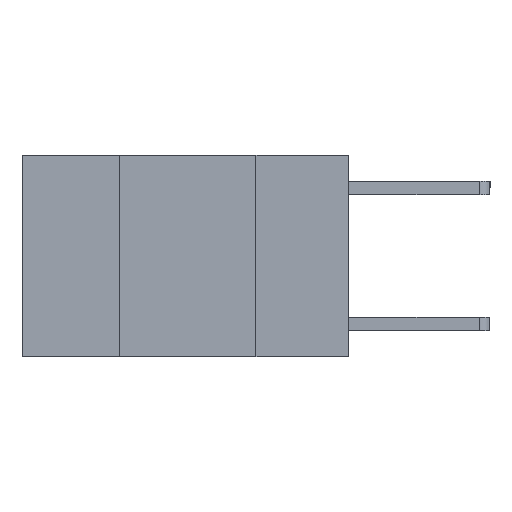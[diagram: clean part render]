
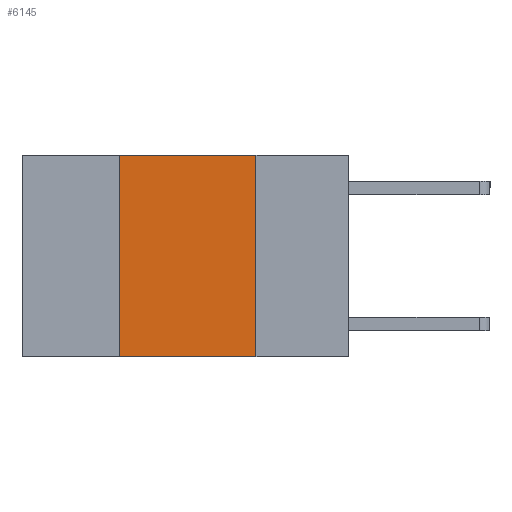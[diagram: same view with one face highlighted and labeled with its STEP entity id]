
A CAD part, left-side view. The second image highlights one B-rep face of the part: STEP entity #6145.
In plain terms, the highlighted planar face has unit normal (-1, 0, 0).
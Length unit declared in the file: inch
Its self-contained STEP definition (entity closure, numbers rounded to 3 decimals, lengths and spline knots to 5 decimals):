
#148 = VECTOR ( 'NONE', #10862, 39.37008 ) ;
#499 = EDGE_CURVE ( 'NONE', #9650, #7800, #9865, .T. ) ;
#1142 = CARTESIAN_POINT ( 'NONE',  ( 0., 0.17, 0. ) ) ;
#1620 = CARTESIAN_POINT ( 'NONE',  ( 0., 0.6, -0.37 ) ) ;
#1632 = VERTEX_POINT ( 'NONE', #6149 ) ;
#1659 = ORIENTED_EDGE ( 'NONE', *, *, #4590, .F. ) ;
#1723 = EDGE_LOOP ( 'NONE', ( #9367, #6712, #1659, #10635 ) ) ;
#2183 = DIRECTION ( 'NONE',  ( 0., -1., 0. ) ) ;
#2272 = PLANE ( 'NONE',  #5442 ) ;
#2622 = DIRECTION ( 'NONE',  ( 0., -1., 0. ) ) ;
#2800 = LINE ( 'NONE', #5513, #9042 ) ;
#3132 = CARTESIAN_POINT ( 'NONE',  ( 0., 0.6, 0. ) ) ;
#3229 = CARTESIAN_POINT ( 'NONE',  ( 0., 0.42, 0. ) ) ;
#4013 = DIRECTION ( 'NONE',  ( 1., 0., 0. ) ) ;
#4117 = CARTESIAN_POINT ( 'NONE',  ( 0., 0.6, 0. ) ) ;
#4304 = EDGE_CURVE ( 'NONE', #10488, #1632, #5051, .T. ) ;
#4462 = CARTESIAN_POINT ( 'NONE',  ( 0., 0.42, -0.37 ) ) ;
#4590 = EDGE_CURVE ( 'NONE', #10488, #9650, #9282, .T. ) ;
#5051 = LINE ( 'NONE', #1620, #5869 ) ;
#5442 = AXIS2_PLACEMENT_3D ( 'NONE', #4117, #4013, #6684 ) ;
#5513 = CARTESIAN_POINT ( 'NONE',  ( 0., 0.17, 0. ) ) ;
#5869 = VECTOR ( 'NONE', #2622, 39.37008 ) ;
#6145 = ADVANCED_FACE ( 'NONE', ( #9051 ), #2272, .F. ) ;
#6149 = CARTESIAN_POINT ( 'NONE',  ( 0., 0.17, -0.37 ) ) ;
#6684 = DIRECTION ( 'NONE',  ( 0., 0., -1. ) ) ;
#6712 = ORIENTED_EDGE ( 'NONE', *, *, #499, .F. ) ;
#6808 = EDGE_CURVE ( 'NONE', #7800, #1632, #2800, .T. ) ;
#7800 = VERTEX_POINT ( 'NONE', #1142 ) ;
#7968 = DIRECTION ( 'NONE',  ( 0., 0., -1. ) ) ;
#9040 = CARTESIAN_POINT ( 'NONE',  ( 0., 0.42, 0. ) ) ;
#9042 = VECTOR ( 'NONE', #7968, 39.37008 ) ;
#9051 = FACE_OUTER_BOUND ( 'NONE', #1723, .T. ) ;
#9282 = LINE ( 'NONE', #3229, #148 ) ;
#9367 = ORIENTED_EDGE ( 'NONE', *, *, #6808, .F. ) ;
#9650 = VERTEX_POINT ( 'NONE', #9040 ) ;
#9865 = LINE ( 'NONE', #3132, #10808 ) ;
#10488 = VERTEX_POINT ( 'NONE', #4462 ) ;
#10635 = ORIENTED_EDGE ( 'NONE', *, *, #4304, .T. ) ;
#10808 = VECTOR ( 'NONE', #2183, 39.37008 ) ;
#10862 = DIRECTION ( 'NONE',  ( 0., 0., 1. ) ) ;
